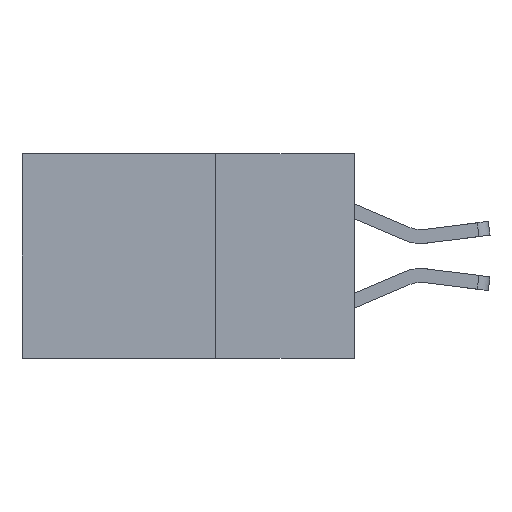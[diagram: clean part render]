
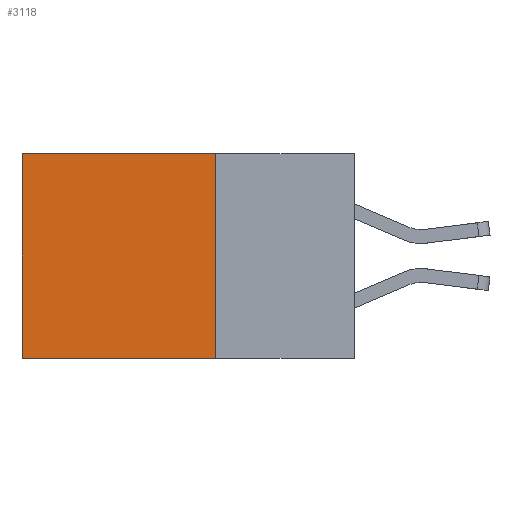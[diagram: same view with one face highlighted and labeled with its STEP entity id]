
A CAD part, left-side view. The second image highlights one B-rep face of the part: STEP entity #3118.
In plain terms, the highlighted planar face has unit normal (-1, 0, 0).
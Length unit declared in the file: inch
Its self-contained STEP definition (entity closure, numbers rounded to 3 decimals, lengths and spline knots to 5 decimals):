
#659 = EDGE_CURVE ( 'NONE', #2781, #7674, #6103, .T. ) ;
#1123 = DIRECTION ( 'NONE',  ( 0., 0., -1. ) ) ;
#1208 = VECTOR ( 'NONE', #2549, 39.37008 ) ;
#1219 = CARTESIAN_POINT ( 'NONE',  ( 0.298, 0.25, 0. ) ) ;
#1972 = ORIENTED_EDGE ( 'NONE', *, *, #3650, .F. ) ;
#2549 = DIRECTION ( 'NONE',  ( 0., 0., -1. ) ) ;
#2781 = VERTEX_POINT ( 'NONE', #1219 ) ;
#3118 = ADVANCED_FACE ( 'NONE', ( #6215 ), #5218, .F. ) ;
#3292 = DIRECTION ( 'NONE',  ( 0., 1., 0. ) ) ;
#3554 = CARTESIAN_POINT ( 'NONE',  ( 0.298, 0.25, 0. ) ) ;
#3650 = EDGE_CURVE ( 'NONE', #2781, #5389, #7916, .T. ) ;
#3666 = AXIS2_PLACEMENT_3D ( 'NONE', #3554, #9425, #4417 ) ;
#3690 = CARTESIAN_POINT ( 'NONE',  ( 0.298, 0.25, -0.37 ) ) ;
#4417 = DIRECTION ( 'NONE',  ( 0., 0., -1. ) ) ;
#4751 = CARTESIAN_POINT ( 'NONE',  ( 0.298, 0.6, 0. ) ) ;
#5218 = PLANE ( 'NONE',  #3666 ) ;
#5389 = VERTEX_POINT ( 'NONE', #10835 ) ;
#5506 = EDGE_LOOP ( 'NONE', ( #7210, #9959, #1972, #9297 ) ) ;
#6103 = LINE ( 'NONE', #9175, #10287 ) ;
#6122 = LINE ( 'NONE', #6160, #10574 ) ;
#6131 = CARTESIAN_POINT ( 'NONE',  ( 0.298, 0.6, -0.37 ) ) ;
#6160 = CARTESIAN_POINT ( 'NONE',  ( 0.298, 0.6, 0. ) ) ;
#6215 = FACE_OUTER_BOUND ( 'NONE', #5506, .T. ) ;
#7210 = ORIENTED_EDGE ( 'NONE', *, *, #10602, .T. ) ;
#7674 = VERTEX_POINT ( 'NONE', #4751 ) ;
#7916 = LINE ( 'NONE', #10102, #1208 ) ;
#8735 = DIRECTION ( 'NONE',  ( 0., 1., 0. ) ) ;
#9175 = CARTESIAN_POINT ( 'NONE',  ( 0.298, 0.25, 0. ) ) ;
#9297 = ORIENTED_EDGE ( 'NONE', *, *, #659, .T. ) ;
#9425 = DIRECTION ( 'NONE',  ( 1., 0., 0. ) ) ;
#9777 = VECTOR ( 'NONE', #8735, 39.37008 ) ;
#9959 = ORIENTED_EDGE ( 'NONE', *, *, #10696, .F. ) ;
#10040 = VERTEX_POINT ( 'NONE', #6131 ) ;
#10042 = LINE ( 'NONE', #3690, #9777 ) ;
#10102 = CARTESIAN_POINT ( 'NONE',  ( 0.298, 0.25, 0. ) ) ;
#10287 = VECTOR ( 'NONE', #3292, 39.37008 ) ;
#10574 = VECTOR ( 'NONE', #1123, 39.37008 ) ;
#10602 = EDGE_CURVE ( 'NONE', #7674, #10040, #6122, .T. ) ;
#10696 = EDGE_CURVE ( 'NONE', #5389, #10040, #10042, .T. ) ;
#10835 = CARTESIAN_POINT ( 'NONE',  ( 0.298, 0.25, -0.37 ) ) ;
